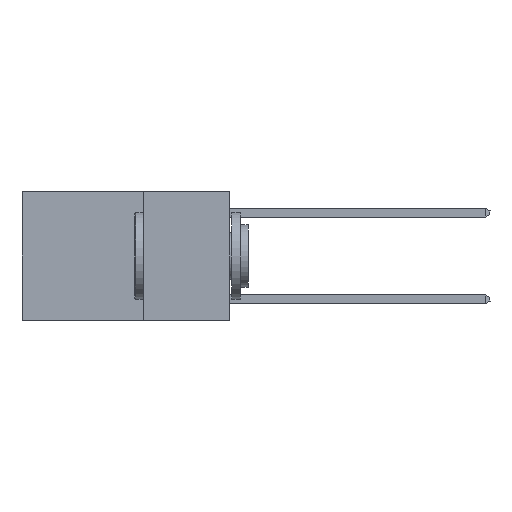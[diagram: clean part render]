
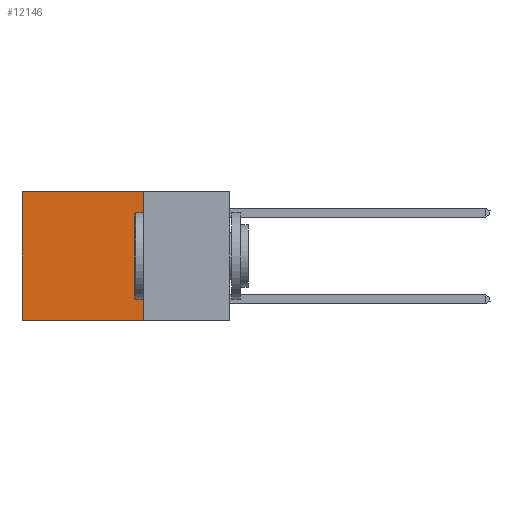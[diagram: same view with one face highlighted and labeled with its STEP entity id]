
A CAD part, left-side view. The second image highlights one B-rep face of the part: STEP entity #12146.
In plain terms, the highlighted planar face has unit normal (-1, 0, 0).
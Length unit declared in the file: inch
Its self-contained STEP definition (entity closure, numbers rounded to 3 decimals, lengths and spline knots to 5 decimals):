
#777 = LINE ( 'NONE', #1934, #5833 ) ;
#913 = DIRECTION ( 'NONE',  ( 0., 1., 0. ) ) ;
#1934 = CARTESIAN_POINT ( 'NONE',  ( 0.2625, 0.25, 0. ) ) ;
#2254 = LINE ( 'NONE', #11632, #12822 ) ;
#2299 = EDGE_LOOP ( 'NONE', ( #8136, #10521, #6756, #4808 ) ) ;
#3151 = DIRECTION ( 'NONE',  ( 0., 1., 0. ) ) ;
#3473 = LINE ( 'NONE', #8602, #8026 ) ;
#4362 = VERTEX_POINT ( 'NONE', #10936 ) ;
#4558 = CARTESIAN_POINT ( 'NONE',  ( 0.2625, 0.6, 0. ) ) ;
#4808 = ORIENTED_EDGE ( 'NONE', *, *, #8063, .T. ) ;
#4825 = DIRECTION ( 'NONE',  ( 1., 0., 0. ) ) ;
#5221 = VERTEX_POINT ( 'NONE', #9539 ) ;
#5231 = EDGE_CURVE ( 'NONE', #11185, #5221, #5511, .T. ) ;
#5253 = CARTESIAN_POINT ( 'NONE',  ( 0.2625, 0.25, 0. ) ) ;
#5511 = LINE ( 'NONE', #5253, #9020 ) ;
#5833 = VECTOR ( 'NONE', #913, 39.37008 ) ;
#5852 = DIRECTION ( 'NONE',  ( 0., 0., -1. ) ) ;
#6477 = EDGE_CURVE ( 'NONE', #5221, #4362, #2254, .T. ) ;
#6756 = ORIENTED_EDGE ( 'NONE', *, *, #5231, .F. ) ;
#7821 = EDGE_CURVE ( 'NONE', #8381, #4362, #3473, .T. ) ;
#8026 = VECTOR ( 'NONE', #10675, 39.37008 ) ;
#8063 = EDGE_CURVE ( 'NONE', #11185, #8381, #777, .T. ) ;
#8136 = ORIENTED_EDGE ( 'NONE', *, *, #7821, .T. ) ;
#8381 = VERTEX_POINT ( 'NONE', #4558 ) ;
#8602 = CARTESIAN_POINT ( 'NONE',  ( 0.2625, 0.6, 0. ) ) ;
#9020 = VECTOR ( 'NONE', #9670, 39.37008 ) ;
#9046 = AXIS2_PLACEMENT_3D ( 'NONE', #11886, #4825, #5852 ) ;
#9057 = FACE_OUTER_BOUND ( 'NONE', #2299, .T. ) ;
#9539 = CARTESIAN_POINT ( 'NONE',  ( 0.2625, 0.25, -0.37 ) ) ;
#9670 = DIRECTION ( 'NONE',  ( 0., 0., -1. ) ) ;
#10444 = CARTESIAN_POINT ( 'NONE',  ( 0.2625, 0.25, 0. ) ) ;
#10521 = ORIENTED_EDGE ( 'NONE', *, *, #6477, .F. ) ;
#10675 = DIRECTION ( 'NONE',  ( 0., 0., -1. ) ) ;
#10936 = CARTESIAN_POINT ( 'NONE',  ( 0.2625, 0.6, -0.37 ) ) ;
#10985 = PLANE ( 'NONE',  #9046 ) ;
#11185 = VERTEX_POINT ( 'NONE', #10444 ) ;
#11632 = CARTESIAN_POINT ( 'NONE',  ( 0.2625, 0.25, -0.37 ) ) ;
#11886 = CARTESIAN_POINT ( 'NONE',  ( 0.2625, 0.25, 0. ) ) ;
#12146 = ADVANCED_FACE ( 'NONE', ( #9057 ), #10985, .F. ) ;
#12822 = VECTOR ( 'NONE', #3151, 39.37008 ) ;
